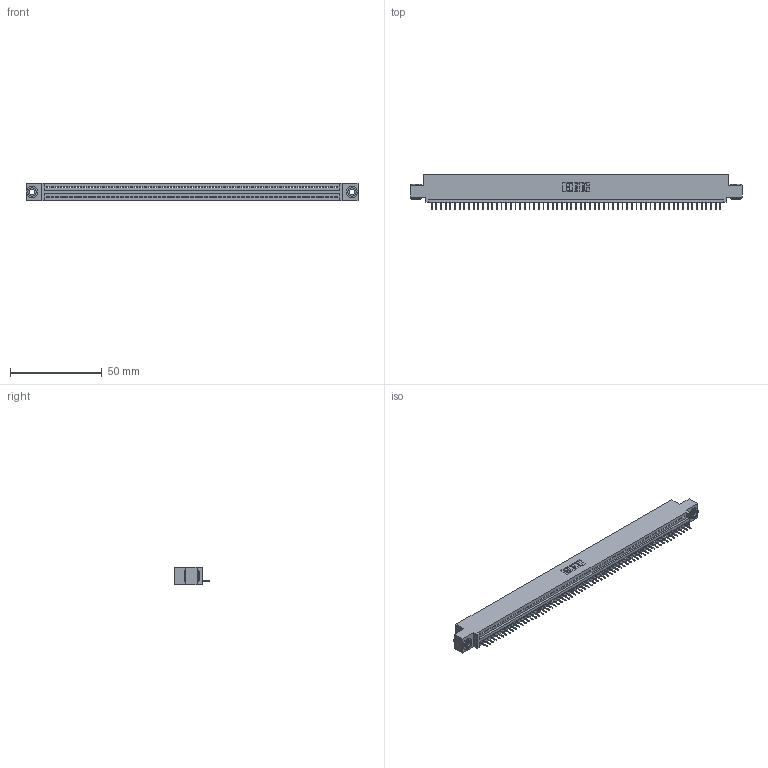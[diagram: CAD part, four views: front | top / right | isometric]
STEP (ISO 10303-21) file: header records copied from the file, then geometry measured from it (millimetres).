
FILE_DESCRIPTION (( 'STEP AP203' ), '1' );
FILE_NAME ('345-063-524-403.STEP', '2019-10-11T10:08:49', ( '' ), ( '' ), 'SwSTEP 2.0', 'SolidWorks 2016', '' );
FILE_SCHEMA (( 'CONFIG_CONTROL_DESIGN' ));
Length unit declared in the file: inch
Products named in the file (4): 345-292-001_345-293-124; 345 Part_0.110 Offset - 0.156 Dia-TH; 345-250-002_345-250-002-102; 345-063-524-403
Assembly tree (66 placements, depth 2):
  345-063-524-403
    345 Part_0.110 Offset - 0.156 Dia-TH
    345-292-001_345-293-124  x63
    345-250-002_345-250-002-102  x2
Bounding box: 181.23 x 19.35 x 9.4 mm (x, y, z)
Volume: 17082.5 mm3; surface area: 22487.2 mm2
Topology: 66 solids, 66 shells, 4074 faces, 11769 edges, 7590 vertices
Faces by surface type: plane 2992, cylinder 1074, cone 8
Entity records: 45444 total; most frequent: CARTESIAN_POINT 7848, ORIENTED_EDGE 7838, DIRECTION 6855, EDGE_CURVE 3919, LINE 3515, VECTOR 3515, VERTEX_POINT 2606, AXIS2_PLACEMENT_3D 1670
